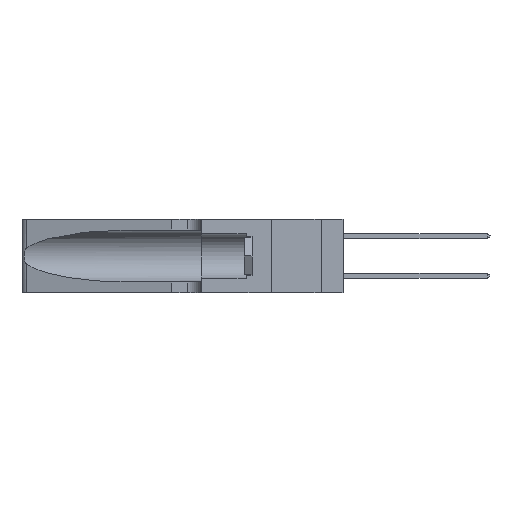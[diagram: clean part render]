
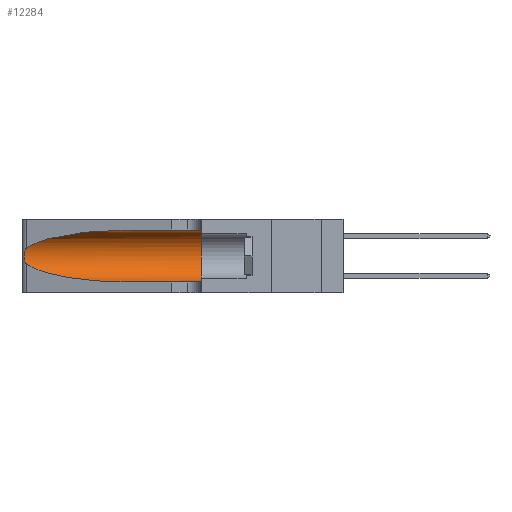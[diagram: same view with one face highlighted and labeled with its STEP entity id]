
A CAD part, left-side view. The second image highlights one B-rep face of the part: STEP entity #12284.
In plain terms, the highlighted cylindrical face has radius 3.308 mm (diameter 6.617 mm), a partial arc.
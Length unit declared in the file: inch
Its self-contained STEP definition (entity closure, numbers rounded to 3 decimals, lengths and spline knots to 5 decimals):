
#1233 = CARTESIAN_POINT ( 'NONE',  ( 0.25639, 1.23186, 0.15144 ) ) ;
#1386 = CARTESIAN_POINT ( 'NONE',  ( 0.25789, 1.23486, 0.15765 ) ) ;
#1929 = ORIENTED_EDGE ( 'NONE', *, *, #23475, .T. ) ;
#2516 = ORIENTED_EDGE ( 'NONE', *, *, #5673, .T. ) ;
#2868 = CARTESIAN_POINT ( 'NONE',  ( 0.25487, 1.22718, 0.14631 ) ) ;
#3012 = CARTESIAN_POINT ( 'NONE',  ( 0.18966, 0.96281, 0.05475 ) ) ;
#5286 = CARTESIAN_POINT ( 'NONE',  ( 0.25854, 1.2359, 0.20912 ) ) ;
#5673 = EDGE_CURVE ( 'NONE', #26572, #26169, #36413, .T. ) ;
#8530 = EDGE_CURVE ( 'NONE', #40734, #10784, #35849, .T. ) ;
#9276 = CARTESIAN_POINT ( 'NONE',  ( 0.25487, 1.22718, 0.22369 ) ) ;
#10580 = EDGE_CURVE ( 'NONE', #26169, #40734, #29180, .T. ) ;
#10649 = CARTESIAN_POINT ( 'NONE',  ( 0.1305, 1.61858, 0.31525 ) ) ;
#10784 = VERTEX_POINT ( 'NONE', #20611 ) ;
#11712 = DIRECTION ( 'NONE',  ( 0., 0., -1. ) ) ;
#11786 = CARTESIAN_POINT ( 'NONE',  ( 0.26018, 1.23835, 0.19895 ) ) ;
#11884 = ORIENTED_EDGE ( 'NONE', *, *, #34681, .F. ) ;
#12284 = ADVANCED_FACE ( 'NONE', ( #43860 ), #27531, .F. ) ;
#12324 = VECTOR ( 'NONE', #21118, 39.37008 ) ;
#12482 = AXIS2_PLACEMENT_3D ( 'NONE', #15204, #35721, #11712 ) ;
#12559 = CARTESIAN_POINT ( 'NONE',  ( 0.25487, 1.22718, 0.22369 ) ) ;
#13182 = ORIENTED_EDGE ( 'NONE', *, *, #39621, .F. ) ;
#13337 = CARTESIAN_POINT ( 'NONE',  ( 0.2373, 1.15595, 0.08982 ) ) ;
#13846 = CARTESIAN_POINT ( 'NONE',  ( 0.1305, 0.35, 0.31525 ) ) ;
#15016 = LINE ( 'NONE', #10649, #12324 ) ;
#15177 = AXIS2_PLACEMENT_3D ( 'NONE', #33476, #43823, #19146 ) ;
#15204 = CARTESIAN_POINT ( 'NONE',  ( 0.1305, 1.61858, 0.185 ) ) ;
#17152 = CIRCLE ( 'NONE', #15177, 0.13025 ) ;
#17248 = CARTESIAN_POINT ( 'NONE',  ( 0.25487, 1.22718, 0.14631 ) ) ;
#17403 = CARTESIAN_POINT ( 'NONE',  ( 0.1305, 1.61858, 0.05475 ) ) ;
#17524 = ORIENTED_EDGE ( 'NONE', *, *, #8530, .T. ) ;
#18734 = CARTESIAN_POINT ( 'NONE',  ( 0.26075, 1.23896, 0.19203 ) ) ;
#19039 = CARTESIAN_POINT ( 'NONE',  ( 0.25555, 1.22993, 0.14849 ) ) ;
#19146 = DIRECTION ( 'NONE',  ( 0., 0., 1. ) ) ;
#19229 = CARTESIAN_POINT ( 'NONE',  ( 0.2373, 1.15595, 0.28018 ) ) ;
#19546 = LINE ( 'NONE', #17403, #33140 ) ;
#19691 = CARTESIAN_POINT ( 'NONE',  ( 0.18966, 0.96281, 0.31525 ) ) ;
#20611 = CARTESIAN_POINT ( 'NONE',  ( 0.1305, 0.72297, 0.05475 ) ) ;
#21104 = ORIENTED_EDGE ( 'NONE', *, *, #10580, .T. ) ;
#21118 = DIRECTION ( 'NONE',  ( 0., -1., 0. ) ) ;
#22395 = CARTESIAN_POINT ( 'NONE',  ( 0.1305, 0.72297, 0.31525 ) ) ;
#23475 = EDGE_CURVE ( 'NONE', #10784, #37145, #19546, .T. ) ;
#24717 = VERTEX_POINT ( 'NONE', #13846 ) ;
#26169 = VERTEX_POINT ( 'NONE', #9276 ) ;
#26572 = VERTEX_POINT ( 'NONE', #22395 ) ;
#27531 = CYLINDRICAL_SURFACE ( 'NONE', #12482, 0.13025 ) ;
#28711 = CARTESIAN_POINT ( 'NONE',  ( 0.25487, 1.22718, 0.22369 ) ) ;
#28766 = EDGE_LOOP ( 'NONE', ( #2516, #21104, #17524, #1929, #13182, #11884 ) ) ;
#28970 = CARTESIAN_POINT ( 'NONE',  ( 0.25856, 1.23593, 0.16098 ) ) ;
#29180 = B_SPLINE_CURVE_WITH_KNOTS ( 'NONE', 3,
 ( #28711, #35697, #41460, #34626, #5286, #11786, #18734, #29439, #36400, #28970, #1386, #1233, #19039, #29602 ),
 .UNSPECIFIED., .F., .F.,
 ( 4, 2, 2, 2, 2, 2, 4 ),
 ( 0., 0.00027, 0.00053, 0.00107, 0.0016, 0.00187, 0.00214 ),
 .UNSPECIFIED. ) ;
#29349 = CARTESIAN_POINT ( 'NONE',  ( 0.1305, 0.35, 0.05475 ) ) ;
#29439 = CARTESIAN_POINT ( 'NONE',  ( 0.26075, 1.23896, 0.178 ) ) ;
#29602 = CARTESIAN_POINT ( 'NONE',  ( 0.25487, 1.22718, 0.14631 ) ) ;
#31546 = CARTESIAN_POINT ( 'NONE',  ( 0.1305, 0.72297, 0.05475 ) ) ;
#33140 = VECTOR ( 'NONE', #37693, 39.37008 ) ;
#33476 = CARTESIAN_POINT ( 'NONE',  ( 0.1305, 0.35, 0.185 ) ) ;
#34626 = CARTESIAN_POINT ( 'NONE',  ( 0.25787, 1.23484, 0.2124 ) ) ;
#34681 = EDGE_CURVE ( 'NONE', #26572, #24717, #15016, .T. ) ;
#35697 = CARTESIAN_POINT ( 'NONE',  ( 0.25555, 1.22994, 0.2215 ) ) ;
#35721 = DIRECTION ( 'NONE',  ( 0., -1., 0. ) ) ;
#35849 =( BOUNDED_CURVE ( )  B_SPLINE_CURVE ( 3, ( #2868, #13337, #3012, #31546 ),
 .UNSPECIFIED., .F., .F. ) 
 B_SPLINE_CURVE_WITH_KNOTS ( ( 4, 4 ),
 ( 3.44316, 4.71239 ),
 .UNSPECIFIED. ) 
 CURVE ( )  GEOMETRIC_REPRESENTATION_ITEM ( )  RATIONAL_B_SPLINE_CURVE ( ( 1., 0.87, 0.87, 1. ) ) 
 REPRESENTATION_ITEM ( '' )  );
#36400 = CARTESIAN_POINT ( 'NONE',  ( 0.26017, 1.23833, 0.17102 ) ) ;
#36413 =( BOUNDED_CURVE ( )  B_SPLINE_CURVE ( 3, ( #40402, #19691, #19229, #12559 ),
 .UNSPECIFIED., .F., .F. ) 
 B_SPLINE_CURVE_WITH_KNOTS ( ( 4, 4 ),
 ( 1.5708, 2.84003 ),
 .UNSPECIFIED. ) 
 CURVE ( )  GEOMETRIC_REPRESENTATION_ITEM ( )  RATIONAL_B_SPLINE_CURVE ( ( 1., 0.87, 0.87, 1. ) ) 
 REPRESENTATION_ITEM ( '' )  );
#37145 = VERTEX_POINT ( 'NONE', #29349 ) ;
#37693 = DIRECTION ( 'NONE',  ( 0., -1., 0. ) ) ;
#39621 = EDGE_CURVE ( 'NONE', #24717, #37145, #17152, .T. ) ;
#40402 = CARTESIAN_POINT ( 'NONE',  ( 0.1305, 0.72297, 0.31525 ) ) ;
#40734 = VERTEX_POINT ( 'NONE', #17248 ) ;
#41460 = CARTESIAN_POINT ( 'NONE',  ( 0.25639, 1.23184, 0.21858 ) ) ;
#43823 = DIRECTION ( 'NONE',  ( 0., 1., 0. ) ) ;
#43860 = FACE_OUTER_BOUND ( 'NONE', #28766, .T. ) ;
